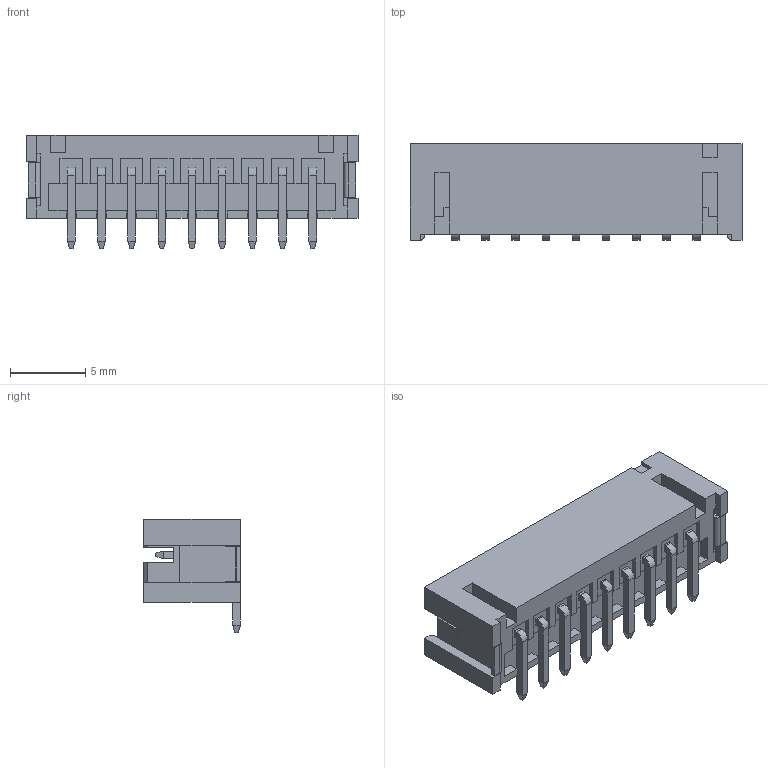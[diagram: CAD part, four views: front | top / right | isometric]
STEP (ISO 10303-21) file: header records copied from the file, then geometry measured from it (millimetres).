
FILE_DESCRIPTION (( 'STEP AP203' ), '1' );
FILE_NAME ('140-509-417-011.STEP', '2020-03-31T20:04:41', ( '' ), ( '' ), 'SwSTEP 2.0', 'SolidWorks 2016', '' );
FILE_SCHEMA (( 'CONFIG_CONTROL_DESIGN' ));
Length unit declared in the file: millimetre
Products named in the file (4): V SMT Pad; 140-509-417-011; V SMT Contact; V SMT Housing_509
Assembly tree (12 placements, depth 2):
  140-509-417-011
    V SMT Housing_509
    V SMT Contact  x9
    V SMT Pad  x2
Bounding box: 22 x 6.4 x 7.5 mm (x, y, z)
Volume: 325.6 mm3; surface area: 1174.4 mm2
Topology: 12 solids, 12 shells, 442 faces, 1112 edges, 690 vertices
Faces by surface type: plane 420, cylinder 22
Entity records: 8794 total; most frequent: CARTESIAN_POINT 1465, ORIENTED_EDGE 1448, DIRECTION 1266, EDGE_CURVE 724, LINE 716, VECTOR 716, VERTEX_POINT 474, AXIS2_PLACEMENT_3D 275
